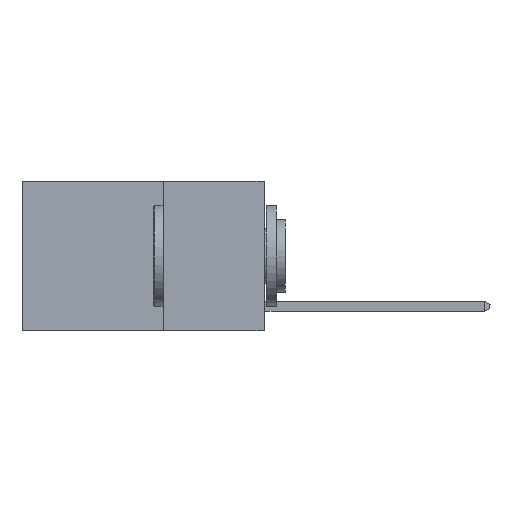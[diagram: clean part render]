
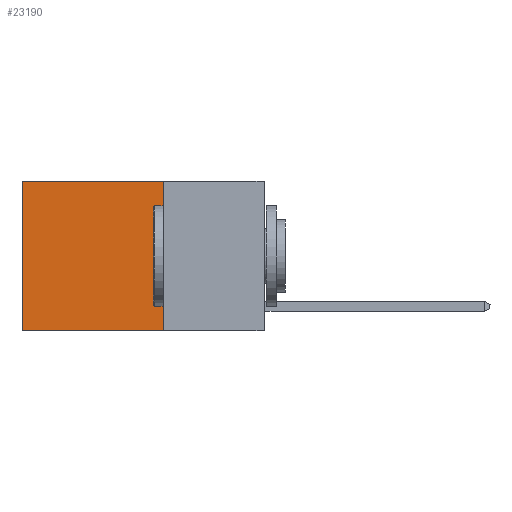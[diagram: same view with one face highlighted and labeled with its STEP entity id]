
A CAD part, left-side view. The second image highlights one B-rep face of the part: STEP entity #23190.
In plain terms, the highlighted planar face has unit normal (-1, 0, 0).
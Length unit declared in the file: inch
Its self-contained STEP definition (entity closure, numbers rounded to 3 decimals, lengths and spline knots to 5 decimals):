
#275 = EDGE_CURVE ( 'NONE', #26408, #2545, #9154, .T. ) ;
#498 = LINE ( 'NONE', #10727, #12995 ) ;
#919 = ORIENTED_EDGE ( 'NONE', *, *, #3406, .F. ) ;
#978 = CARTESIAN_POINT ( 'NONE',  ( 0.2625, 0.6, 0. ) ) ;
#2545 = VERTEX_POINT ( 'NONE', #17543 ) ;
#3406 = EDGE_CURVE ( 'NONE', #7409, #26408, #25746, .T. ) ;
#4671 = FACE_OUTER_BOUND ( 'NONE', #15046, .T. ) ;
#6641 = CARTESIAN_POINT ( 'NONE',  ( 0.2625, 0.25, 0. ) ) ;
#6868 = DIRECTION ( 'NONE',  ( 0., 1., 0. ) ) ;
#7153 = VECTOR ( 'NONE', #6868, 39.37008 ) ;
#7226 = VERTEX_POINT ( 'NONE', #978 ) ;
#7409 = VERTEX_POINT ( 'NONE', #22894 ) ;
#9154 = LINE ( 'NONE', #15578, #7153 ) ;
#9213 = DIRECTION ( 'NONE',  ( 0., 0., -1. ) ) ;
#10463 = ORIENTED_EDGE ( 'NONE', *, *, #12506, .T. ) ;
#10727 = CARTESIAN_POINT ( 'NONE',  ( 0.2625, 0.6, 0. ) ) ;
#11030 = LINE ( 'NONE', #27847, #25908 ) ;
#11041 = ORIENTED_EDGE ( 'NONE', *, *, #275, .F. ) ;
#11388 = AXIS2_PLACEMENT_3D ( 'NONE', #6641, #13493, #9213 ) ;
#11574 = VECTOR ( 'NONE', #27871, 39.37008 ) ;
#12506 = EDGE_CURVE ( 'NONE', #7409, #7226, #11030, .T. ) ;
#12995 = VECTOR ( 'NONE', #19999, 39.37008 ) ;
#13493 = DIRECTION ( 'NONE',  ( 1., 0., 0. ) ) ;
#15046 = EDGE_LOOP ( 'NONE', ( #16896, #11041, #919, #10463 ) ) ;
#15578 = CARTESIAN_POINT ( 'NONE',  ( 0.2625, 0.25, -0.37 ) ) ;
#16574 = EDGE_CURVE ( 'NONE', #7226, #2545, #498, .T. ) ;
#16896 = ORIENTED_EDGE ( 'NONE', *, *, #16574, .T. ) ;
#17543 = CARTESIAN_POINT ( 'NONE',  ( 0.2625, 0.6, -0.37 ) ) ;
#19999 = DIRECTION ( 'NONE',  ( 0., 0., -1. ) ) ;
#21759 = PLANE ( 'NONE',  #11388 ) ;
#22894 = CARTESIAN_POINT ( 'NONE',  ( 0.2625, 0.25, 0. ) ) ;
#23190 = ADVANCED_FACE ( 'NONE', ( #4671 ), #21759, .F. ) ;
#25327 = CARTESIAN_POINT ( 'NONE',  ( 0.2625, 0.25, -0.37 ) ) ;
#25746 = LINE ( 'NONE', #26171, #11574 ) ;
#25908 = VECTOR ( 'NONE', #26015, 39.37008 ) ;
#26015 = DIRECTION ( 'NONE',  ( 0., 1., 0. ) ) ;
#26171 = CARTESIAN_POINT ( 'NONE',  ( 0.2625, 0.25, 0. ) ) ;
#26408 = VERTEX_POINT ( 'NONE', #25327 ) ;
#27847 = CARTESIAN_POINT ( 'NONE',  ( 0.2625, 0.25, 0. ) ) ;
#27871 = DIRECTION ( 'NONE',  ( 0., 0., -1. ) ) ;
